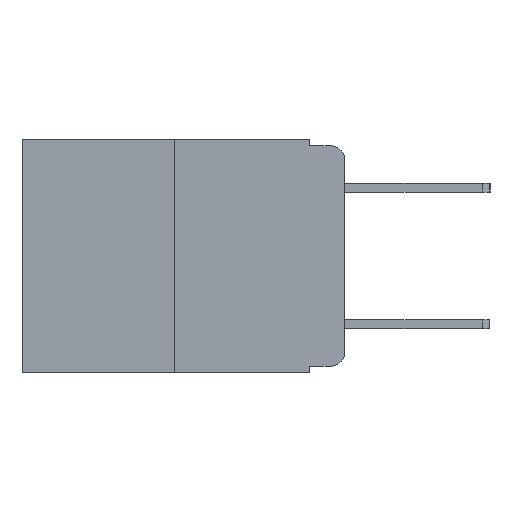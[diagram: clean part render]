
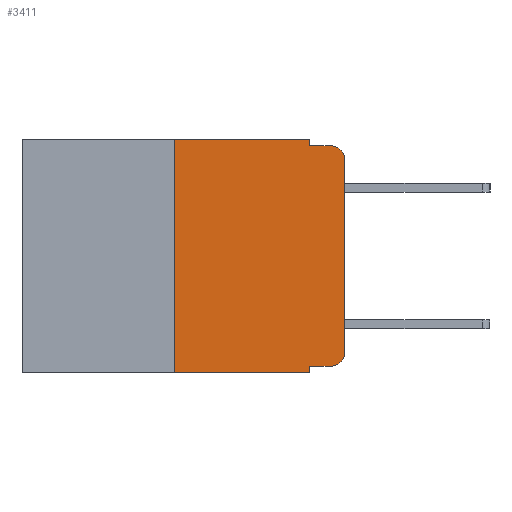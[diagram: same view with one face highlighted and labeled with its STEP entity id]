
A CAD part, left-side view. The second image highlights one B-rep face of the part: STEP entity #3411.
In plain terms, the highlighted planar face has unit normal (-1, 0, 0).
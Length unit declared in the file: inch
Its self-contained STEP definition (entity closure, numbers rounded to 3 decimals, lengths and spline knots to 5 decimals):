
#193 = EDGE_CURVE ( 'NONE', #8342, #6231, #4184, .T. ) ;
#371 = VECTOR ( 'NONE', #10674, 39.37008 ) ;
#778 = LINE ( 'NONE', #2891, #8317 ) ;
#863 = ORIENTED_EDGE ( 'NONE', *, *, #5356, .F. ) ;
#1188 = VERTEX_POINT ( 'NONE', #1683 ) ;
#1211 = EDGE_LOOP ( 'NONE', ( #7955, #8646, #863, #5861, #4545, #9185, #9977, #8486, #10772, #11094 ) ) ;
#1323 = CIRCLE ( 'NONE', #9938, 0.02 ) ;
#1457 = DIRECTION ( 'NONE',  ( -1., 0., 0. ) ) ;
#1478 = VERTEX_POINT ( 'NONE', #9777 ) ;
#1683 = CARTESIAN_POINT ( 'NONE',  ( 0., 0.051, -0.01 ) ) ;
#1785 = VECTOR ( 'NONE', #8794, 39.37008 ) ;
#2580 = VERTEX_POINT ( 'NONE', #9843 ) ;
#2717 = CARTESIAN_POINT ( 'NONE',  ( 0., 0., -0.313 ) ) ;
#2891 = CARTESIAN_POINT ( 'NONE',  ( 0., 0.051, 0. ) ) ;
#3084 = VECTOR ( 'NONE', #11021, 39.37008 ) ;
#3087 = DIRECTION ( 'NONE',  ( 0., -1., 0. ) ) ;
#3411 = ADVANCED_FACE ( 'NONE', ( #8730 ), #9008, .F. ) ;
#3536 = VERTEX_POINT ( 'NONE', #8631 ) ;
#3543 = VERTEX_POINT ( 'NONE', #11178 ) ;
#3923 = CARTESIAN_POINT ( 'NONE',  ( 0., 0.02, -0.03 ) ) ;
#4184 = LINE ( 'NONE', #7544, #8361 ) ;
#4545 = ORIENTED_EDGE ( 'NONE', *, *, #9867, .F. ) ;
#4562 = EDGE_CURVE ( 'NONE', #3536, #1478, #6067, .T. ) ;
#4668 = EDGE_CURVE ( 'NONE', #6584, #8342, #1323, .T. ) ;
#4787 = EDGE_CURVE ( 'NONE', #3536, #6584, #6592, .T. ) ;
#4809 = EDGE_CURVE ( 'NONE', #2580, #1188, #778, .T. ) ;
#4824 = EDGE_CURVE ( 'NONE', #3543, #7460, #10277, .T. ) ;
#4972 = DIRECTION ( 'NONE',  ( 0., 0., 1. ) ) ;
#5018 = DIRECTION ( 'NONE',  ( 0., 0., -1. ) ) ;
#5065 = CARTESIAN_POINT ( 'NONE',  ( 0., 0.051, -0.01 ) ) ;
#5105 = CARTESIAN_POINT ( 'NONE',  ( 0., 0.473, -0.343 ) ) ;
#5336 = EDGE_CURVE ( 'NONE', #6231, #7959, #10255, .T. ) ;
#5356 = EDGE_CURVE ( 'NONE', #1188, #7959, #6039, .T. ) ;
#5447 = EDGE_CURVE ( 'NONE', #3543, #1478, #8653, .T. ) ;
#5694 = CARTESIAN_POINT ( 'NONE',  ( 0., 0.02, -0.01 ) ) ;
#5861 = ORIENTED_EDGE ( 'NONE', *, *, #4809, .F. ) ;
#5920 = DIRECTION ( 'NONE',  ( 0., 0., -1. ) ) ;
#6039 = LINE ( 'NONE', #5065, #9805 ) ;
#6067 = LINE ( 'NONE', #10292, #3084 ) ;
#6231 = VERTEX_POINT ( 'NONE', #7285 ) ;
#6323 = AXIS2_PLACEMENT_3D ( 'NONE', #9020, #11658, #11674 ) ;
#6437 = VECTOR ( 'NONE', #3087, 39.37008 ) ;
#6584 = VERTEX_POINT ( 'NONE', #9080 ) ;
#6592 = LINE ( 'NONE', #6743, #10512 ) ;
#6743 = CARTESIAN_POINT ( 'NONE',  ( 0., 0.051, -0.333 ) ) ;
#7110 = LINE ( 'NONE', #10990, #1785 ) ;
#7285 = CARTESIAN_POINT ( 'NONE',  ( 0., 0., -0.03 ) ) ;
#7435 = CARTESIAN_POINT ( 'NONE',  ( 0., 0.02, -0.313 ) ) ;
#7460 = VERTEX_POINT ( 'NONE', #11313 ) ;
#7544 = CARTESIAN_POINT ( 'NONE',  ( 0., 0., 0. ) ) ;
#7955 = ORIENTED_EDGE ( 'NONE', *, *, #193, .T. ) ;
#7959 = VERTEX_POINT ( 'NONE', #5694 ) ;
#8263 = DIRECTION ( 'NONE',  ( 0., 0., -1. ) ) ;
#8317 = VECTOR ( 'NONE', #5920, 39.37008 ) ;
#8342 = VERTEX_POINT ( 'NONE', #2717 ) ;
#8361 = VECTOR ( 'NONE', #4972, 39.37008 ) ;
#8431 = DIRECTION ( 'NONE',  ( 0., -1., 0. ) ) ;
#8486 = ORIENTED_EDGE ( 'NONE', *, *, #4562, .F. ) ;
#8631 = CARTESIAN_POINT ( 'NONE',  ( 0., 0.051, -0.333 ) ) ;
#8646 = ORIENTED_EDGE ( 'NONE', *, *, #5336, .T. ) ;
#8653 = LINE ( 'NONE', #5105, #6437 ) ;
#8730 = FACE_OUTER_BOUND ( 'NONE', #1211, .T. ) ;
#8794 = DIRECTION ( 'NONE',  ( 0., -1., 0. ) ) ;
#9008 = PLANE ( 'NONE',  #6323 ) ;
#9020 = CARTESIAN_POINT ( 'NONE',  ( 0., 0.473, 0. ) ) ;
#9080 = CARTESIAN_POINT ( 'NONE',  ( 0., 0.02, -0.333 ) ) ;
#9185 = ORIENTED_EDGE ( 'NONE', *, *, #4824, .F. ) ;
#9777 = CARTESIAN_POINT ( 'NONE',  ( 0., 0.051, -0.343 ) ) ;
#9805 = VECTOR ( 'NONE', #11370, 39.37008 ) ;
#9843 = CARTESIAN_POINT ( 'NONE',  ( 0., 0.051, 0. ) ) ;
#9867 = EDGE_CURVE ( 'NONE', #7460, #2580, #7110, .T. ) ;
#9885 = DIRECTION ( 'NONE',  ( -1., 0., 0. ) ) ;
#9938 = AXIS2_PLACEMENT_3D ( 'NONE', #7435, #1457, #8263 ) ;
#9977 = ORIENTED_EDGE ( 'NONE', *, *, #5447, .T. ) ;
#10251 = AXIS2_PLACEMENT_3D ( 'NONE', #3923, #9885, #5018 ) ;
#10255 = CIRCLE ( 'NONE', #10251, 0.02 ) ;
#10277 = LINE ( 'NONE', #11357, #371 ) ;
#10292 = CARTESIAN_POINT ( 'NONE',  ( 0., 0.051, 0. ) ) ;
#10512 = VECTOR ( 'NONE', #8431, 39.37008 ) ;
#10674 = DIRECTION ( 'NONE',  ( 0., 0., 1. ) ) ;
#10772 = ORIENTED_EDGE ( 'NONE', *, *, #4787, .T. ) ;
#10990 = CARTESIAN_POINT ( 'NONE',  ( 0., 0.473, 0. ) ) ;
#11021 = DIRECTION ( 'NONE',  ( 0., 0., -1. ) ) ;
#11094 = ORIENTED_EDGE ( 'NONE', *, *, #4668, .T. ) ;
#11178 = CARTESIAN_POINT ( 'NONE',  ( 0., 0.25, -0.343 ) ) ;
#11313 = CARTESIAN_POINT ( 'NONE',  ( 0., 0.25, 0. ) ) ;
#11357 = CARTESIAN_POINT ( 'NONE',  ( 0., 0.25, 0. ) ) ;
#11370 = DIRECTION ( 'NONE',  ( 0., -1., 0. ) ) ;
#11658 = DIRECTION ( 'NONE',  ( 1., 0., 0. ) ) ;
#11674 = DIRECTION ( 'NONE',  ( 0., 0., -1. ) ) ;
